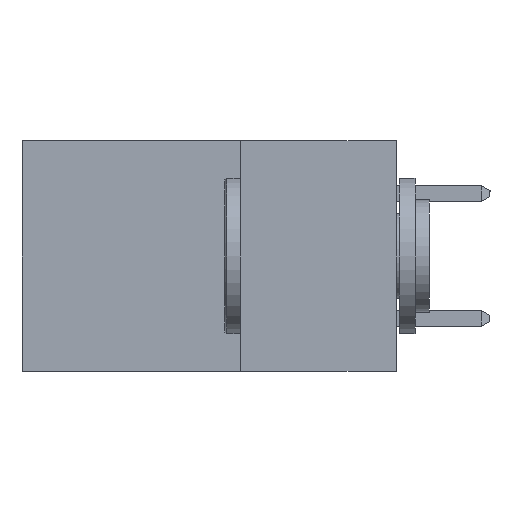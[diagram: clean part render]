
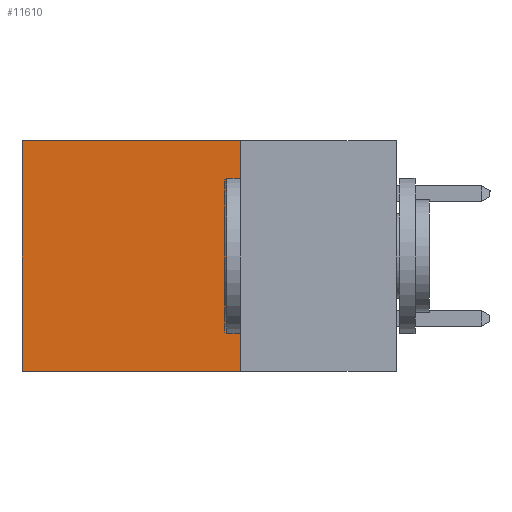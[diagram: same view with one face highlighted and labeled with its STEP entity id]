
A CAD part, left-side view. The second image highlights one B-rep face of the part: STEP entity #11610.
In plain terms, the highlighted planar face has unit normal (-1, 0, 0).
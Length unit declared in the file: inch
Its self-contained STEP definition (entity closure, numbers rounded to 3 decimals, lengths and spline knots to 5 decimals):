
#341 = ORIENTED_EDGE ( 'NONE', *, *, #7126, .F. ) ;
#478 = LINE ( 'NONE', #12819, #13008 ) ;
#815 = PLANE ( 'NONE',  #4393 ) ;
#1967 = LINE ( 'NONE', #5714, #11476 ) ;
#2373 = VECTOR ( 'NONE', #15380, 39.37008 ) ;
#2814 = ORIENTED_EDGE ( 'NONE', *, *, #3780, .T. ) ;
#3013 = EDGE_CURVE ( 'NONE', #8071, #14436, #11400, .T. ) ;
#3780 = EDGE_CURVE ( 'NONE', #11579, #8071, #478, .T. ) ;
#4393 = AXIS2_PLACEMENT_3D ( 'NONE', #11953, #10961, #14770 ) ;
#5185 = CARTESIAN_POINT ( 'NONE',  ( 0.2615, 0.25, -0.37 ) ) ;
#5714 = CARTESIAN_POINT ( 'NONE',  ( 0.2615, 0.25, -0.37 ) ) ;
#6040 = VECTOR ( 'NONE', #15830, 39.37008 ) ;
#6959 = CARTESIAN_POINT ( 'NONE',  ( 0.2615, 0.25, 0. ) ) ;
#7126 = EDGE_CURVE ( 'NONE', #11579, #14509, #1967, .T. ) ;
#7809 = CARTESIAN_POINT ( 'NONE',  ( 0.2615, 0.6, -0.37 ) ) ;
#8071 = VERTEX_POINT ( 'NONE', #15129 ) ;
#8128 = DIRECTION ( 'NONE',  ( 0., 0., -1. ) ) ;
#8354 = LINE ( 'NONE', #13428, #6040 ) ;
#8920 = DIRECTION ( 'NONE',  ( 0., 1., 0. ) ) ;
#10961 = DIRECTION ( 'NONE',  ( 1., 0., 0. ) ) ;
#11400 = LINE ( 'NONE', #7809, #2373 ) ;
#11476 = VECTOR ( 'NONE', #8128, 39.37008 ) ;
#11579 = VERTEX_POINT ( 'NONE', #6959 ) ;
#11610 = ADVANCED_FACE ( 'NONE', ( #12189 ), #815, .F. ) ;
#11953 = CARTESIAN_POINT ( 'NONE',  ( 0.2615, 0.25, -0.37 ) ) ;
#12189 = FACE_OUTER_BOUND ( 'NONE', #14052, .T. ) ;
#12330 = ORIENTED_EDGE ( 'NONE', *, *, #3013, .T. ) ;
#12819 = CARTESIAN_POINT ( 'NONE',  ( 0.2615, 0.25, 0. ) ) ;
#12842 = CARTESIAN_POINT ( 'NONE',  ( 0.2615, 0.6, -0.37 ) ) ;
#13008 = VECTOR ( 'NONE', #8920, 39.37008 ) ;
#13359 = EDGE_CURVE ( 'NONE', #14509, #14436, #8354, .T. ) ;
#13428 = CARTESIAN_POINT ( 'NONE',  ( 0.2615, 0.25, -0.37 ) ) ;
#14052 = EDGE_LOOP ( 'NONE', ( #12330, #14270, #341, #2814 ) ) ;
#14270 = ORIENTED_EDGE ( 'NONE', *, *, #13359, .F. ) ;
#14436 = VERTEX_POINT ( 'NONE', #12842 ) ;
#14509 = VERTEX_POINT ( 'NONE', #5185 ) ;
#14770 = DIRECTION ( 'NONE',  ( 0., 0., -1. ) ) ;
#15129 = CARTESIAN_POINT ( 'NONE',  ( 0.2615, 0.6, 0. ) ) ;
#15380 = DIRECTION ( 'NONE',  ( 0., 0., -1. ) ) ;
#15830 = DIRECTION ( 'NONE',  ( 0., 1., 0. ) ) ;
